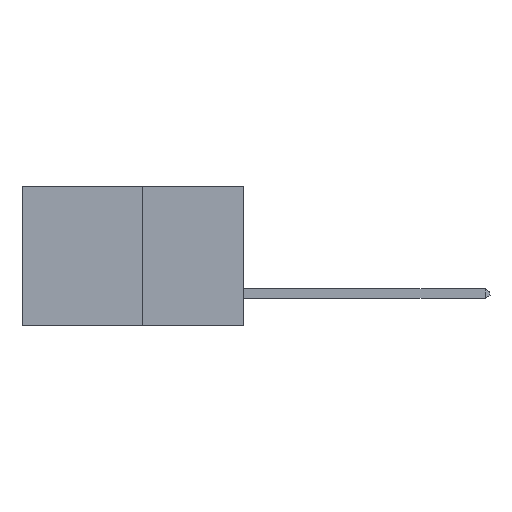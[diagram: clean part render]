
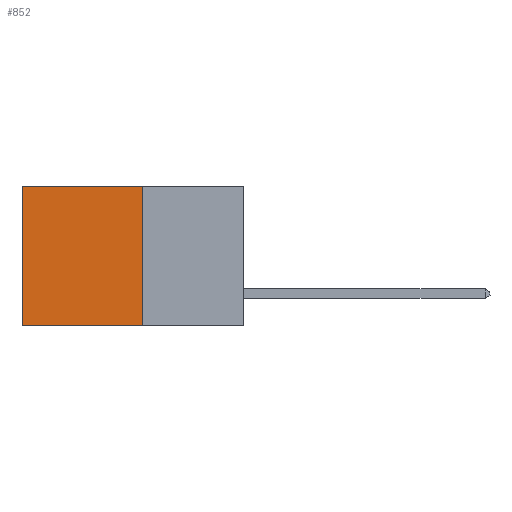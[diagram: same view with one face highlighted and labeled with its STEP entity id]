
A CAD part, left-side view. The second image highlights one B-rep face of the part: STEP entity #852.
In plain terms, the highlighted planar face has unit normal (-1, 0, 0).
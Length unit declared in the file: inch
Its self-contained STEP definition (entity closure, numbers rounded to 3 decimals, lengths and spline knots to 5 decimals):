
#561 = CARTESIAN_POINT ( 'NONE',  ( 0.277, 0.59, -0.37 ) ) ;
#639 = ORIENTED_EDGE ( 'NONE', *, *, #4037, .F. ) ;
#852 = ADVANCED_FACE ( 'NONE', ( #11429 ), #8921, .F. ) ;
#1012 = CARTESIAN_POINT ( 'NONE',  ( 0.277, 0.27, -0.37 ) ) ;
#1231 = LINE ( 'NONE', #561, #10668 ) ;
#2269 = CARTESIAN_POINT ( 'NONE',  ( 0.277, 0.27, 0. ) ) ;
#2439 = VECTOR ( 'NONE', #3454, 39.37008 ) ;
#2714 = ORIENTED_EDGE ( 'NONE', *, *, #10155, .T. ) ;
#3298 = VECTOR ( 'NONE', #11677, 39.37008 ) ;
#3454 = DIRECTION ( 'NONE',  ( 0., 1., 0. ) ) ;
#4037 = EDGE_CURVE ( 'NONE', #6859, #9813, #5728, .T. ) ;
#4953 = LINE ( 'NONE', #7112, #2439 ) ;
#5041 = CARTESIAN_POINT ( 'NONE',  ( 0.277, 0.59, 0. ) ) ;
#5728 = LINE ( 'NONE', #8682, #3298 ) ;
#6259 = VERTEX_POINT ( 'NONE', #5041 ) ;
#6698 = ORIENTED_EDGE ( 'NONE', *, *, #10394, .F. ) ;
#6859 = VERTEX_POINT ( 'NONE', #1012 ) ;
#7112 = CARTESIAN_POINT ( 'NONE',  ( 0.277, 0.27, 0. ) ) ;
#7347 = CARTESIAN_POINT ( 'NONE',  ( 0.277, 0.27, -0.37 ) ) ;
#7493 = EDGE_LOOP ( 'NONE', ( #11374, #639, #6698, #2714 ) ) ;
#7925 = VERTEX_POINT ( 'NONE', #2269 ) ;
#8326 = LINE ( 'NONE', #10011, #10094 ) ;
#8682 = CARTESIAN_POINT ( 'NONE',  ( 0.277, 0.27, -0.37 ) ) ;
#8905 = DIRECTION ( 'NONE',  ( 0., 0., -1. ) ) ;
#8921 = PLANE ( 'NONE',  #11777 ) ;
#9321 = DIRECTION ( 'NONE',  ( 1., 0., 0. ) ) ;
#9333 = DIRECTION ( 'NONE',  ( 0., 0., -1. ) ) ;
#9813 = VERTEX_POINT ( 'NONE', #11162 ) ;
#10011 = CARTESIAN_POINT ( 'NONE',  ( 0.277, 0.27, -0.37 ) ) ;
#10094 = VECTOR ( 'NONE', #10941, 39.37008 ) ;
#10155 = EDGE_CURVE ( 'NONE', #7925, #6259, #4953, .T. ) ;
#10394 = EDGE_CURVE ( 'NONE', #7925, #6859, #8326, .T. ) ;
#10668 = VECTOR ( 'NONE', #8905, 39.37008 ) ;
#10865 = EDGE_CURVE ( 'NONE', #6259, #9813, #1231, .T. ) ;
#10941 = DIRECTION ( 'NONE',  ( 0., 0., -1. ) ) ;
#11162 = CARTESIAN_POINT ( 'NONE',  ( 0.277, 0.59, -0.37 ) ) ;
#11374 = ORIENTED_EDGE ( 'NONE', *, *, #10865, .T. ) ;
#11429 = FACE_OUTER_BOUND ( 'NONE', #7493, .T. ) ;
#11677 = DIRECTION ( 'NONE',  ( 0., 1., 0. ) ) ;
#11777 = AXIS2_PLACEMENT_3D ( 'NONE', #7347, #9321, #9333 ) ;
